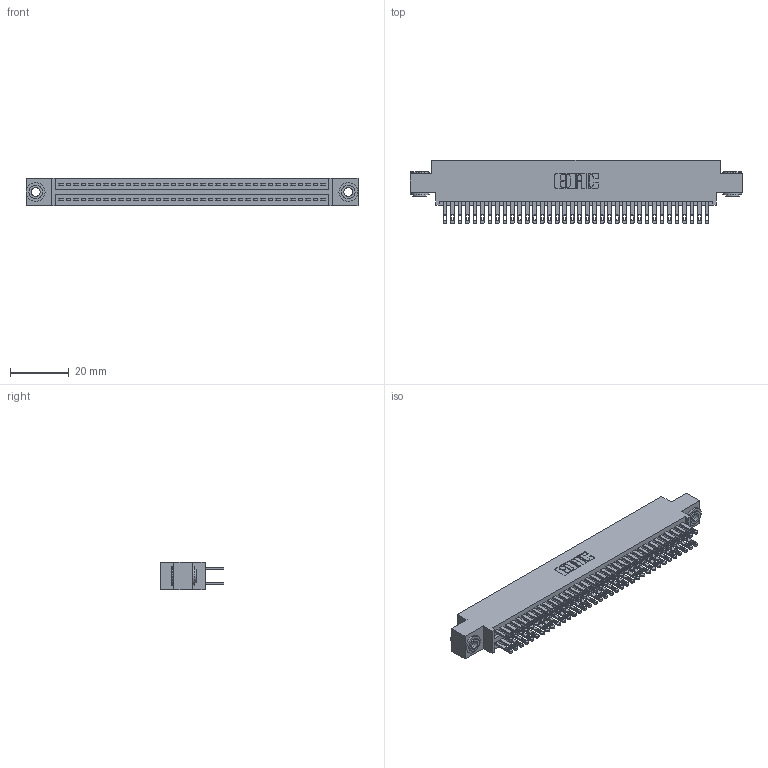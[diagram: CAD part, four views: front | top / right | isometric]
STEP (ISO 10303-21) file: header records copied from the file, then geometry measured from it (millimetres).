
FILE_DESCRIPTION (( 'STEP AP203' ), '1' );
FILE_NAME ('345-072-500-803.STEP', '2019-10-31T02:22:16', ( '' ), ( '' ), 'SwSTEP 2.0', 'SolidWorks 2016', '' );
FILE_SCHEMA (( 'CONFIG_CONTROL_DESIGN' ));
Length unit declared in the file: inch
Products named in the file (4): 345-072-500-803; 345-250-002_345-250-002-102; 345-292-001_345-293-100; 345 Part_0.170 Offset - 0.156 Dia-TH
Assembly tree (75 placements, depth 2):
  345-072-500-803
    345 Part_0.170 Offset - 0.156 Dia-TH
    345-292-001_345-293-100  x72
    345-250-002_345-250-002-102  x2
Bounding box: 112.65 x 21.51 x 9.4 mm (x, y, z)
Volume: 11013.2 mm3; surface area: 17245.8 mm2
Topology: 75 solids, 75 shells, 3480 faces, 10581 edges, 7050 vertices
Faces by surface type: plane 2038, cylinder 1434, cone 8
Entity records: 29766 total; most frequent: CARTESIAN_POINT 4971, ORIENTED_EDGE 4898, DIRECTION 4423, EDGE_CURVE 2449, VECTOR 2145, LINE 2145, VERTEX_POINT 1630, AXIS2_PLACEMENT_3D 1139
